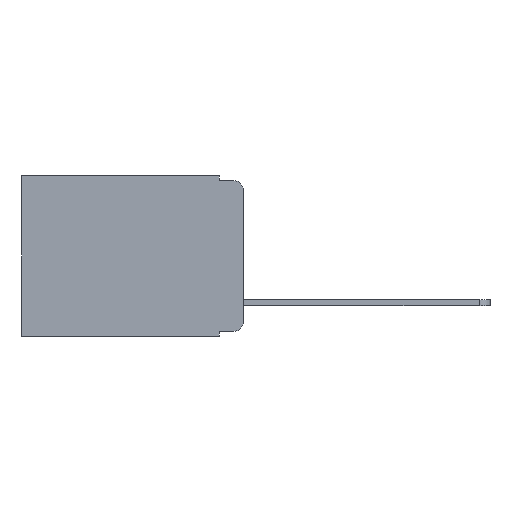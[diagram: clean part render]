
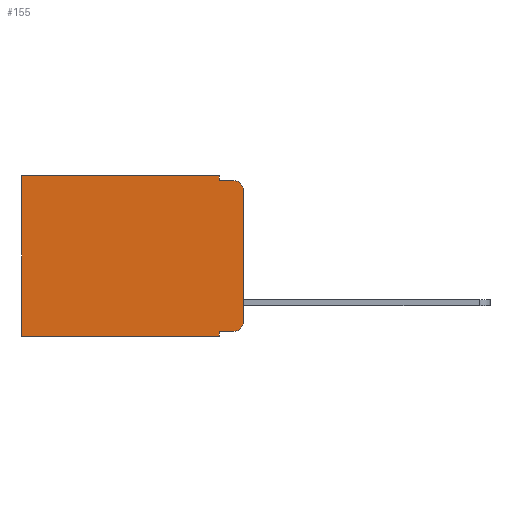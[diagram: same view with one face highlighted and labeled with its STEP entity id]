
A CAD part, left-side view. The second image highlights one B-rep face of the part: STEP entity #155.
In plain terms, the highlighted planar face has unit normal (-1, 0, 0).
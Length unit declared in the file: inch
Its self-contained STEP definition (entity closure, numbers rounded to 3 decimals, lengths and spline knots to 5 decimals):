
#3 = LINE ( 'NONE', #8683, #7999 ) ;
#155 = ADVANCED_FACE ( 'NONE', ( #8221 ), #2119, .F. ) ;
#216 = DIRECTION ( 'NONE',  ( 0., -1., 0. ) ) ;
#254 = VERTEX_POINT ( 'NONE', #4711 ) ;
#281 = VERTEX_POINT ( 'NONE', #6209 ) ;
#500 = VERTEX_POINT ( 'NONE', #7742 ) ;
#501 = EDGE_CURVE ( 'NONE', #281, #500, #3, .T. ) ;
#502 = AXIS2_PLACEMENT_3D ( 'NONE', #9718, #8318, #9656 ) ;
#606 = LINE ( 'NONE', #7059, #8212 ) ;
#645 = EDGE_CURVE ( 'NONE', #4053, #6182, #3239, .T. ) ;
#726 = VERTEX_POINT ( 'NONE', #7777 ) ;
#773 = ORIENTED_EDGE ( 'NONE', *, *, #3095, .F. ) ;
#991 = VERTEX_POINT ( 'NONE', #2097 ) ;
#992 = DIRECTION ( 'NONE',  ( 1., 0., 0. ) ) ;
#1078 = VERTEX_POINT ( 'NONE', #8424 ) ;
#1236 = DIRECTION ( 'NONE',  ( 0., -1., 0. ) ) ;
#1250 = EDGE_CURVE ( 'NONE', #500, #6854, #606, .T. ) ;
#1529 = LINE ( 'NONE', #9104, #5421 ) ;
#1795 = ORIENTED_EDGE ( 'NONE', *, *, #645, .F. ) ;
#1855 = ORIENTED_EDGE ( 'NONE', *, *, #3836, .T. ) ;
#1859 = ORIENTED_EDGE ( 'NONE', *, *, #8895, .F. ) ;
#1903 = ORIENTED_EDGE ( 'NONE', *, *, #7986, .F. ) ;
#2066 = CARTESIAN_POINT ( 'NONE',  ( 0.298, 0., -0.03 ) ) ;
#2097 = CARTESIAN_POINT ( 'NONE',  ( 0.298, 0.02, -0.01 ) ) ;
#2119 = PLANE ( 'NONE',  #6623 ) ;
#2312 = LINE ( 'NONE', #3779, #7960 ) ;
#2464 = VECTOR ( 'NONE', #7477, 39.37008 ) ;
#2704 = CARTESIAN_POINT ( 'NONE',  ( 0.298, 0.473, -0.343 ) ) ;
#3024 = DIRECTION ( 'NONE',  ( 0., 1., 0. ) ) ;
#3095 = EDGE_CURVE ( 'NONE', #726, #6854, #3375, .T. ) ;
#3180 = ORIENTED_EDGE ( 'NONE', *, *, #6057, .T. ) ;
#3193 = VERTEX_POINT ( 'NONE', #4236 ) ;
#3239 = LINE ( 'NONE', #4437, #8946 ) ;
#3375 = LINE ( 'NONE', #3723, #5575 ) ;
#3471 = DIRECTION ( 'NONE',  ( 0., 0., -1. ) ) ;
#3540 = ORIENTED_EDGE ( 'NONE', *, *, #9343, .F. ) ;
#3561 = LINE ( 'NONE', #6658, #7450 ) ;
#3723 = CARTESIAN_POINT ( 'NONE',  ( 0.298, 0., -0.343 ) ) ;
#3779 = CARTESIAN_POINT ( 'NONE',  ( 0.298, 0.051, 0. ) ) ;
#3807 = CARTESIAN_POINT ( 'NONE',  ( 0.298, 0.02, -0.313 ) ) ;
#3836 = EDGE_CURVE ( 'NONE', #4053, #991, #3964, .T. ) ;
#3964 = CIRCLE ( 'NONE', #502, 0.02 ) ;
#4053 = VERTEX_POINT ( 'NONE', #2066 ) ;
#4162 = DIRECTION ( 'NONE',  ( 0., 0., -1. ) ) ;
#4236 = CARTESIAN_POINT ( 'NONE',  ( 0.298, 0.051, -0.01 ) ) ;
#4338 = ORIENTED_EDGE ( 'NONE', *, *, #1250, .T. ) ;
#4437 = CARTESIAN_POINT ( 'NONE',  ( 0.298, 0., 0. ) ) ;
#4463 = DIRECTION ( 'NONE',  ( 0., 0., -1. ) ) ;
#4524 = DIRECTION ( 'NONE',  ( 0., 0., -1. ) ) ;
#4548 = DIRECTION ( 'NONE',  ( 0., 0., -1. ) ) ;
#4611 = AXIS2_PLACEMENT_3D ( 'NONE', #3807, #8785, #4548 ) ;
#4711 = CARTESIAN_POINT ( 'NONE',  ( 0.298, 0.02, -0.333 ) ) ;
#5421 = VECTOR ( 'NONE', #216, 39.37008 ) ;
#5575 = VECTOR ( 'NONE', #3024, 39.37008 ) ;
#5816 = ORIENTED_EDGE ( 'NONE', *, *, #501, .T. ) ;
#6006 = CARTESIAN_POINT ( 'NONE',  ( 0.298, 0.051, 0. ) ) ;
#6057 = EDGE_CURVE ( 'NONE', #254, #6182, #6819, .T. ) ;
#6164 = ORIENTED_EDGE ( 'NONE', *, *, #6339, .T. ) ;
#6182 = VERTEX_POINT ( 'NONE', #6269 ) ;
#6209 = CARTESIAN_POINT ( 'NONE',  ( 0.298, 0.051, 0. ) ) ;
#6269 = CARTESIAN_POINT ( 'NONE',  ( 0.298, 0., -0.313 ) ) ;
#6339 = EDGE_CURVE ( 'NONE', #1078, #254, #3561, .T. ) ;
#6623 = AXIS2_PLACEMENT_3D ( 'NONE', #7410, #992, #4463 ) ;
#6658 = CARTESIAN_POINT ( 'NONE',  ( 0.298, 0.051, -0.333 ) ) ;
#6819 = CIRCLE ( 'NONE', #4611, 0.02 ) ;
#6854 = VERTEX_POINT ( 'NONE', #2704 ) ;
#7059 = CARTESIAN_POINT ( 'NONE',  ( 0.298, 0.473, 0. ) ) ;
#7410 = CARTESIAN_POINT ( 'NONE',  ( 0.298, 0., 0. ) ) ;
#7450 = VECTOR ( 'NONE', #1236, 39.37008 ) ;
#7477 = DIRECTION ( 'NONE',  ( 0., 0., -1. ) ) ;
#7526 = DIRECTION ( 'NONE',  ( 0., 1., 0. ) ) ;
#7742 = CARTESIAN_POINT ( 'NONE',  ( 0.298, 0.473, 0. ) ) ;
#7777 = CARTESIAN_POINT ( 'NONE',  ( 0.298, 0.051, -0.343 ) ) ;
#7960 = VECTOR ( 'NONE', #4524, 39.37008 ) ;
#7986 = EDGE_CURVE ( 'NONE', #281, #3193, #8296, .T. ) ;
#7999 = VECTOR ( 'NONE', #7526, 39.37008 ) ;
#8212 = VECTOR ( 'NONE', #4162, 39.37008 ) ;
#8221 = FACE_OUTER_BOUND ( 'NONE', #8250, .T. ) ;
#8250 = EDGE_LOOP ( 'NONE', ( #1795, #1855, #1859, #1903, #5816, #4338, #773, #3540, #6164, #3180 ) ) ;
#8296 = LINE ( 'NONE', #6006, #2464 ) ;
#8318 = DIRECTION ( 'NONE',  ( -1., 0., 0. ) ) ;
#8424 = CARTESIAN_POINT ( 'NONE',  ( 0.298, 0.051, -0.333 ) ) ;
#8683 = CARTESIAN_POINT ( 'NONE',  ( 0.298, 0., 0. ) ) ;
#8785 = DIRECTION ( 'NONE',  ( -1., 0., 0. ) ) ;
#8895 = EDGE_CURVE ( 'NONE', #3193, #991, #1529, .T. ) ;
#8946 = VECTOR ( 'NONE', #3471, 39.37008 ) ;
#9104 = CARTESIAN_POINT ( 'NONE',  ( 0.298, 0.051, -0.01 ) ) ;
#9343 = EDGE_CURVE ( 'NONE', #1078, #726, #2312, .T. ) ;
#9656 = DIRECTION ( 'NONE',  ( 0., 0., -1. ) ) ;
#9718 = CARTESIAN_POINT ( 'NONE',  ( 0.298, 0.02, -0.03 ) ) ;
